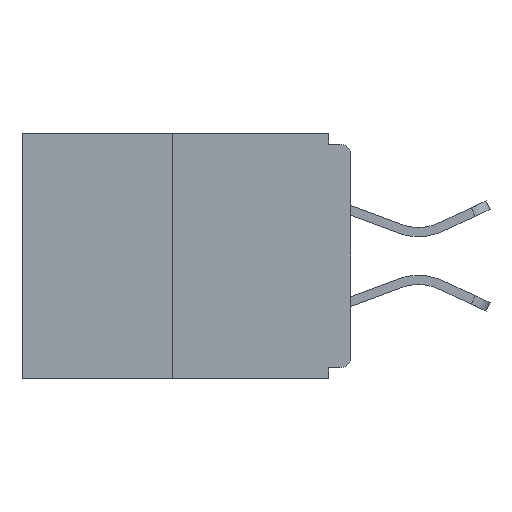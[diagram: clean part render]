
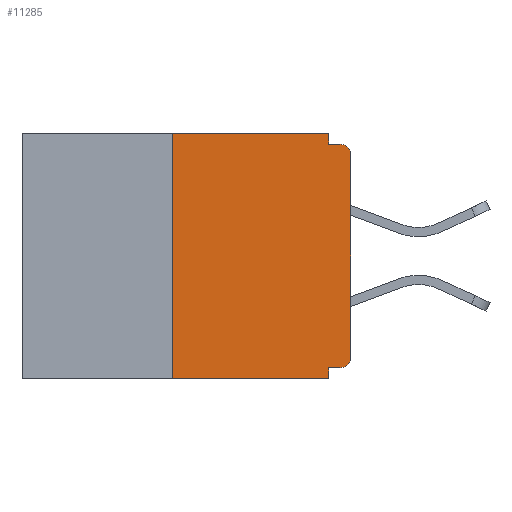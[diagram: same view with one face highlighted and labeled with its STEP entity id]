
A CAD part, left-side view. The second image highlights one B-rep face of the part: STEP entity #11285.
In plain terms, the highlighted planar face has unit normal (-1, 0, 0).
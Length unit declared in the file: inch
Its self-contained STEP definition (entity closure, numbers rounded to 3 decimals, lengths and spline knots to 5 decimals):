
#282 = CARTESIAN_POINT ( 'NONE',  ( 0., 0.25, 0. ) ) ;
#351 = DIRECTION ( 'NONE',  ( 0., 1., 0. ) ) ;
#532 = ORIENTED_EDGE ( 'NONE', *, *, #1600, .T. ) ;
#708 = ORIENTED_EDGE ( 'NONE', *, *, #10144, .T. ) ;
#715 = LINE ( 'NONE', #7249, #11458 ) ;
#1012 = DIRECTION ( 'NONE',  ( 0., 0., -1. ) ) ;
#1133 = VECTOR ( 'NONE', #2426, 39.37008 ) ;
#1164 = ORIENTED_EDGE ( 'NONE', *, *, #4293, .F. ) ;
#1330 = LINE ( 'NONE', #282, #2952 ) ;
#1372 = CARTESIAN_POINT ( 'NONE',  ( 0., 0., 0. ) ) ;
#1600 = EDGE_CURVE ( 'NONE', #11416, #2717, #2646, .T. ) ;
#2037 = DIRECTION ( 'NONE',  ( 0., 0., 1. ) ) ;
#2074 = CARTESIAN_POINT ( 'NONE',  ( 0., 0.031, 0. ) ) ;
#2101 = DIRECTION ( 'NONE',  ( 0., 0., -1. ) ) ;
#2132 = DIRECTION ( 'NONE',  ( 0., 0., -1. ) ) ;
#2278 = DIRECTION ( 'NONE',  ( 0., 0., -1. ) ) ;
#2361 = DIRECTION ( 'NONE',  ( 0., 0., 1. ) ) ;
#2426 = DIRECTION ( 'NONE',  ( 0., -1., 0. ) ) ;
#2578 = VECTOR ( 'NONE', #2361, 39.37008 ) ;
#2646 = CIRCLE ( 'NONE', #9734, 0.015 ) ;
#2717 = VERTEX_POINT ( 'NONE', #10651 ) ;
#2952 = VECTOR ( 'NONE', #2037, 39.37008 ) ;
#3081 = LINE ( 'NONE', #6582, #9477 ) ;
#3104 = CARTESIAN_POINT ( 'NONE',  ( 0., 0.015, -0.328 ) ) ;
#3202 = EDGE_CURVE ( 'NONE', #11416, #10811, #715, .T. ) ;
#3235 = AXIS2_PLACEMENT_3D ( 'NONE', #7435, #4761, #6560 ) ;
#3401 = DIRECTION ( 'NONE',  ( 1., 0., 0. ) ) ;
#3905 = ORIENTED_EDGE ( 'NONE', *, *, #9297, .F. ) ;
#3971 = CARTESIAN_POINT ( 'NONE',  ( 0., 0.031, -0.015 ) ) ;
#4147 = DIRECTION ( 'NONE',  ( 0., -1., 0. ) ) ;
#4293 = EDGE_CURVE ( 'NONE', #8180, #6383, #5986, .T. ) ;
#4576 = EDGE_CURVE ( 'NONE', #6573, #9619, #8275, .T. ) ;
#4761 = DIRECTION ( 'NONE',  ( -1., 0., 0. ) ) ;
#4788 = CARTESIAN_POINT ( 'NONE',  ( 0., 0.015, -0.313 ) ) ;
#4799 = ORIENTED_EDGE ( 'NONE', *, *, #10138, .F. ) ;
#5446 = CARTESIAN_POINT ( 'NONE',  ( 0., 0.46, 0. ) ) ;
#5509 = AXIS2_PLACEMENT_3D ( 'NONE', #5446, #3401, #1012 ) ;
#5831 = CARTESIAN_POINT ( 'NONE',  ( 0., 0.031, -0.343 ) ) ;
#5862 = VECTOR ( 'NONE', #2132, 39.37008 ) ;
#5869 = VERTEX_POINT ( 'NONE', #3971 ) ;
#5895 = LINE ( 'NONE', #7823, #11132 ) ;
#5986 = LINE ( 'NONE', #6814, #1133 ) ;
#6166 = ORIENTED_EDGE ( 'NONE', *, *, #10516, .F. ) ;
#6383 = VERTEX_POINT ( 'NONE', #7570 ) ;
#6464 = CARTESIAN_POINT ( 'NONE',  ( 0., 0.25, -0.343 ) ) ;
#6560 = DIRECTION ( 'NONE',  ( 0., 0., -1. ) ) ;
#6573 = VERTEX_POINT ( 'NONE', #8857 ) ;
#6582 = CARTESIAN_POINT ( 'NONE',  ( 0., 0.46, -0.343 ) ) ;
#6814 = CARTESIAN_POINT ( 'NONE',  ( 0., 0.46, 0. ) ) ;
#6823 = EDGE_CURVE ( 'NONE', #2717, #6573, #8679, .T. ) ;
#7060 = ORIENTED_EDGE ( 'NONE', *, *, #9132, .F. ) ;
#7249 = CARTESIAN_POINT ( 'NONE',  ( 0., 0., -0.328 ) ) ;
#7435 = CARTESIAN_POINT ( 'NONE',  ( 0., 0.015, -0.03 ) ) ;
#7534 = LINE ( 'NONE', #9014, #10384 ) ;
#7570 = CARTESIAN_POINT ( 'NONE',  ( 0., 0.031, 0. ) ) ;
#7823 = CARTESIAN_POINT ( 'NONE',  ( 0., 0., -0.015 ) ) ;
#7888 = VERTEX_POINT ( 'NONE', #5831 ) ;
#8003 = EDGE_LOOP ( 'NONE', ( #1164, #4799, #708, #7060, #8871, #532, #10985, #8880, #3905, #6166 ) ) ;
#8018 = PLANE ( 'NONE',  #5509 ) ;
#8180 = VERTEX_POINT ( 'NONE', #9156 ) ;
#8275 = CIRCLE ( 'NONE', #3235, 0.015 ) ;
#8679 = LINE ( 'NONE', #1372, #2578 ) ;
#8836 = FACE_OUTER_BOUND ( 'NONE', #8003, .T. ) ;
#8857 = CARTESIAN_POINT ( 'NONE',  ( 0., 0., -0.03 ) ) ;
#8871 = ORIENTED_EDGE ( 'NONE', *, *, #3202, .F. ) ;
#8880 = ORIENTED_EDGE ( 'NONE', *, *, #4576, .T. ) ;
#9014 = CARTESIAN_POINT ( 'NONE',  ( 0., 0.031, -0.343 ) ) ;
#9132 = EDGE_CURVE ( 'NONE', #10811, #7888, #7534, .T. ) ;
#9156 = CARTESIAN_POINT ( 'NONE',  ( 0., 0.25, 0. ) ) ;
#9297 = EDGE_CURVE ( 'NONE', #5869, #9619, #5895, .T. ) ;
#9413 = CARTESIAN_POINT ( 'NONE',  ( 0., 0.015, -0.015 ) ) ;
#9477 = VECTOR ( 'NONE', #11067, 39.37008 ) ;
#9619 = VERTEX_POINT ( 'NONE', #9413 ) ;
#9734 = AXIS2_PLACEMENT_3D ( 'NONE', #4788, #11143, #2101 ) ;
#10138 = EDGE_CURVE ( 'NONE', #10544, #8180, #1330, .T. ) ;
#10144 = EDGE_CURVE ( 'NONE', #10544, #7888, #3081, .T. ) ;
#10251 = LINE ( 'NONE', #2074, #5862 ) ;
#10384 = VECTOR ( 'NONE', #2278, 39.37008 ) ;
#10516 = EDGE_CURVE ( 'NONE', #6383, #5869, #10251, .T. ) ;
#10544 = VERTEX_POINT ( 'NONE', #6464 ) ;
#10651 = CARTESIAN_POINT ( 'NONE',  ( 0., 0., -0.313 ) ) ;
#10811 = VERTEX_POINT ( 'NONE', #10822 ) ;
#10822 = CARTESIAN_POINT ( 'NONE',  ( 0., 0.031, -0.328 ) ) ;
#10985 = ORIENTED_EDGE ( 'NONE', *, *, #6823, .T. ) ;
#11067 = DIRECTION ( 'NONE',  ( 0., -1., 0. ) ) ;
#11132 = VECTOR ( 'NONE', #4147, 39.37008 ) ;
#11143 = DIRECTION ( 'NONE',  ( -1., 0., 0. ) ) ;
#11285 = ADVANCED_FACE ( 'NONE', ( #8836 ), #8018, .F. ) ;
#11416 = VERTEX_POINT ( 'NONE', #3104 ) ;
#11458 = VECTOR ( 'NONE', #351, 39.37008 ) ;
